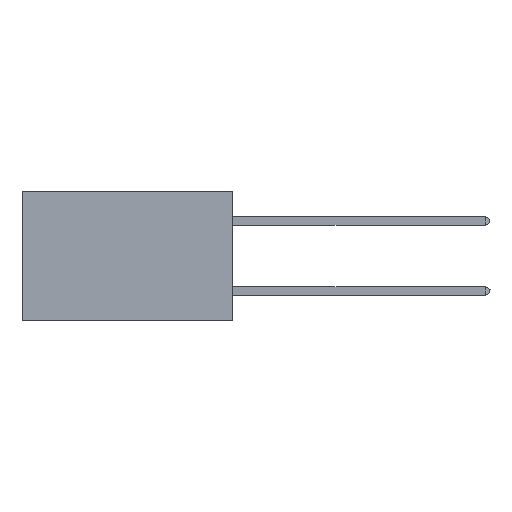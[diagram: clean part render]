
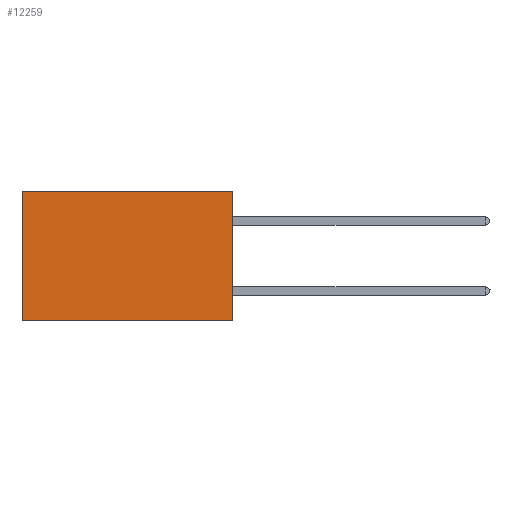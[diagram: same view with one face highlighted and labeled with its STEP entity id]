
A CAD part, left-side view. The second image highlights one B-rep face of the part: STEP entity #12259.
In plain terms, the highlighted planar face has unit normal (-1, 0, 0).
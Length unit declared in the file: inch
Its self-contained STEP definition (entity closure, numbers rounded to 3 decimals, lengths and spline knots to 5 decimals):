
#68 = VECTOR ( 'NONE', #3693, 39.37008 ) ;
#258 = CARTESIAN_POINT ( 'NONE',  ( 0.2875, 0., 0. ) ) ;
#978 = VECTOR ( 'NONE', #9417, 39.37008 ) ;
#1088 = DIRECTION ( 'NONE',  ( 0., 0., -1. ) ) ;
#1213 = DIRECTION ( 'NONE',  ( 0., 0., -1. ) ) ;
#1298 = DIRECTION ( 'NONE',  ( 0., 1., 0. ) ) ;
#1918 = CARTESIAN_POINT ( 'NONE',  ( 0.2875, 0., -0.37 ) ) ;
#2437 = CARTESIAN_POINT ( 'NONE',  ( 0.2875, 0., -0.37 ) ) ;
#2850 = ORIENTED_EDGE ( 'NONE', *, *, #14767, .T. ) ;
#3589 = CARTESIAN_POINT ( 'NONE',  ( 0.2875, 0., 0. ) ) ;
#3693 = DIRECTION ( 'NONE',  ( 0., 1., 0. ) ) ;
#4891 = ORIENTED_EDGE ( 'NONE', *, *, #17483, .T. ) ;
#5388 = CARTESIAN_POINT ( 'NONE',  ( 0.2875, 0., 0. ) ) ;
#5650 = LINE ( 'NONE', #5388, #14118 ) ;
#5767 = LINE ( 'NONE', #3589, #978 ) ;
#7032 = CARTESIAN_POINT ( 'NONE',  ( 0.2875, 0.6, 0. ) ) ;
#8657 = VERTEX_POINT ( 'NONE', #13082 ) ;
#9131 = CARTESIAN_POINT ( 'NONE',  ( 0.2875, 0.6, -0.37 ) ) ;
#9417 = DIRECTION ( 'NONE',  ( 0., 0., -1. ) ) ;
#9688 = EDGE_CURVE ( 'NONE', #15941, #15677, #10539, .T. ) ;
#10066 = ORIENTED_EDGE ( 'NONE', *, *, #9688, .F. ) ;
#10400 = ORIENTED_EDGE ( 'NONE', *, *, #10764, .F. ) ;
#10539 = LINE ( 'NONE', #1918, #68 ) ;
#10764 = EDGE_CURVE ( 'NONE', #12312, #15941, #5767, .T. ) ;
#12259 = ADVANCED_FACE ( 'NONE', ( #15888 ), #14049, .F. ) ;
#12312 = VERTEX_POINT ( 'NONE', #258 ) ;
#12665 = AXIS2_PLACEMENT_3D ( 'NONE', #15526, #18197, #1213 ) ;
#13063 = VECTOR ( 'NONE', #1088, 39.37008 ) ;
#13082 = CARTESIAN_POINT ( 'NONE',  ( 0.2875, 0.6, 0. ) ) ;
#13516 = LINE ( 'NONE', #7032, #13063 ) ;
#14049 = PLANE ( 'NONE',  #12665 ) ;
#14118 = VECTOR ( 'NONE', #1298, 39.37008 ) ;
#14767 = EDGE_CURVE ( 'NONE', #8657, #15677, #13516, .T. ) ;
#15526 = CARTESIAN_POINT ( 'NONE',  ( 0.2875, 0., 0. ) ) ;
#15677 = VERTEX_POINT ( 'NONE', #9131 ) ;
#15888 = FACE_OUTER_BOUND ( 'NONE', #17043, .T. ) ;
#15941 = VERTEX_POINT ( 'NONE', #2437 ) ;
#17043 = EDGE_LOOP ( 'NONE', ( #2850, #10066, #10400, #4891 ) ) ;
#17483 = EDGE_CURVE ( 'NONE', #12312, #8657, #5650, .T. ) ;
#18197 = DIRECTION ( 'NONE',  ( 1., 0., 0. ) ) ;
